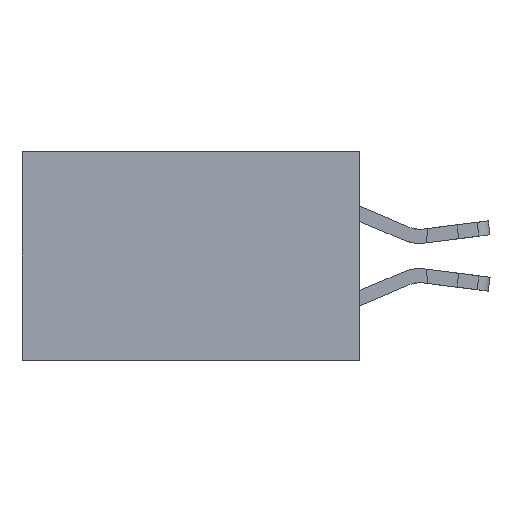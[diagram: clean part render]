
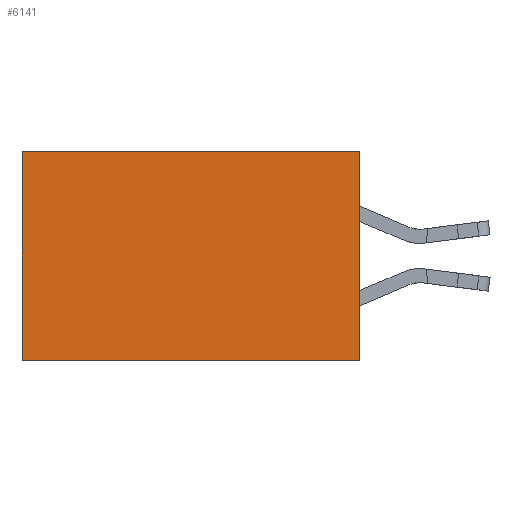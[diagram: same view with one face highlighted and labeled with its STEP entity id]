
A CAD part, left-side view. The second image highlights one B-rep face of the part: STEP entity #6141.
In plain terms, the highlighted planar face has unit normal (-1, 0, 0).
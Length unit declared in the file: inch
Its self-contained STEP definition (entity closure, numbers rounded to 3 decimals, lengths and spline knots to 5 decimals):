
#452 = CARTESIAN_POINT ( 'NONE',  ( 0.2875, 0., 0. ) ) ;
#1347 = EDGE_CURVE ( 'NONE', #24950, #9178, #23178, .T. ) ;
#1526 = FACE_OUTER_BOUND ( 'NONE', #15705, .T. ) ;
#2412 = DIRECTION ( 'NONE',  ( 1., 0., 0. ) ) ;
#4231 = ORIENTED_EDGE ( 'NONE', *, *, #6730, .F. ) ;
#4516 = CARTESIAN_POINT ( 'NONE',  ( 0.2875, 0.6, 0. ) ) ;
#4641 = PLANE ( 'NONE',  #21898 ) ;
#4740 = DIRECTION ( 'NONE',  ( 0., 0., -1. ) ) ;
#6141 = ADVANCED_FACE ( 'NONE', ( #1526 ), #4641, .F. ) ;
#6694 = LINE ( 'NONE', #9941, #24879 ) ;
#6730 = EDGE_CURVE ( 'NONE', #21036, #9178, #7844, .T. ) ;
#7831 = ORIENTED_EDGE ( 'NONE', *, *, #1347, .T. ) ;
#7844 = LINE ( 'NONE', #27732, #8513 ) ;
#8513 = VECTOR ( 'NONE', #16864, 39.37008 ) ;
#9178 = VERTEX_POINT ( 'NONE', #22778 ) ;
#9385 = CARTESIAN_POINT ( 'NONE',  ( 0.2875, 0.6, 0. ) ) ;
#9941 = CARTESIAN_POINT ( 'NONE',  ( 0.2875, 0., 0. ) ) ;
#10686 = ORIENTED_EDGE ( 'NONE', *, *, #19240, .F. ) ;
#11859 = DIRECTION ( 'NONE',  ( 0., 1., 0. ) ) ;
#11935 = DIRECTION ( 'NONE',  ( 0., 0., -1. ) ) ;
#12086 = ORIENTED_EDGE ( 'NONE', *, *, #18777, .T. ) ;
#15705 = EDGE_LOOP ( 'NONE', ( #7831, #4231, #10686, #12086 ) ) ;
#16864 = DIRECTION ( 'NONE',  ( 0., 1., 0. ) ) ;
#16906 = VERTEX_POINT ( 'NONE', #25405 ) ;
#18777 = EDGE_CURVE ( 'NONE', #16906, #24950, #6694, .T. ) ;
#18809 = LINE ( 'NONE', #452, #19801 ) ;
#18853 = VECTOR ( 'NONE', #11935, 39.37008 ) ;
#19240 = EDGE_CURVE ( 'NONE', #16906, #21036, #18809, .T. ) ;
#19587 = DIRECTION ( 'NONE',  ( 0., 0., -1. ) ) ;
#19801 = VECTOR ( 'NONE', #19587, 39.37008 ) ;
#21036 = VERTEX_POINT ( 'NONE', #26177 ) ;
#21898 = AXIS2_PLACEMENT_3D ( 'NONE', #21909, #2412, #4740 ) ;
#21909 = CARTESIAN_POINT ( 'NONE',  ( 0.2875, 0., 0. ) ) ;
#22778 = CARTESIAN_POINT ( 'NONE',  ( 0.2875, 0.6, -0.37 ) ) ;
#23178 = LINE ( 'NONE', #9385, #18853 ) ;
#24879 = VECTOR ( 'NONE', #11859, 39.37008 ) ;
#24950 = VERTEX_POINT ( 'NONE', #4516 ) ;
#25405 = CARTESIAN_POINT ( 'NONE',  ( 0.2875, 0., 0. ) ) ;
#26177 = CARTESIAN_POINT ( 'NONE',  ( 0.2875, 0., -0.37 ) ) ;
#27732 = CARTESIAN_POINT ( 'NONE',  ( 0.2875, 0., -0.37 ) ) ;
